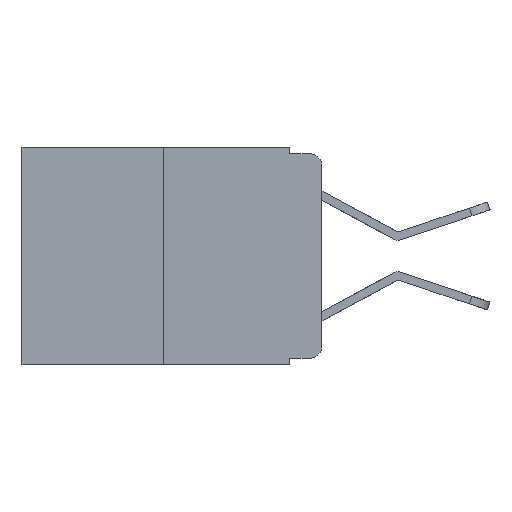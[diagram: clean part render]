
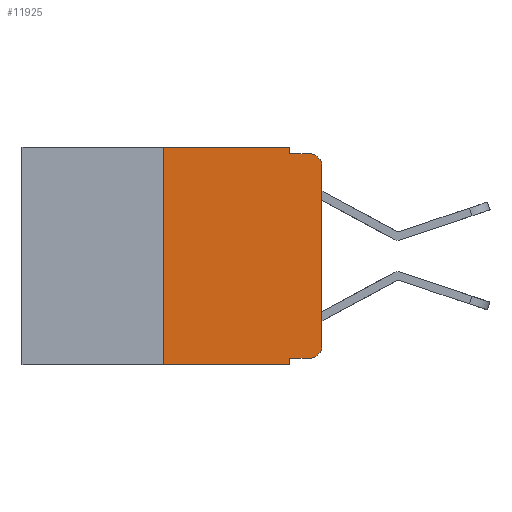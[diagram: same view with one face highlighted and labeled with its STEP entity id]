
A CAD part, left-side view. The second image highlights one B-rep face of the part: STEP entity #11925.
In plain terms, the highlighted planar face has unit normal (-1, 0, 0).
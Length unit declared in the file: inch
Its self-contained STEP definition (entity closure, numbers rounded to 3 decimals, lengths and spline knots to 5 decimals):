
#504 = CARTESIAN_POINT ( 'NONE',  ( 0., 0.02, -0.313 ) ) ;
#676 = DIRECTION ( 'NONE',  ( 0., 0., 1. ) ) ;
#902 = VECTOR ( 'NONE', #6379, 39.37008 ) ;
#942 = LINE ( 'NONE', #8084, #8021 ) ;
#1065 = CARTESIAN_POINT ( 'NONE',  ( 0., 0.051, -0.333 ) ) ;
#1176 = ORIENTED_EDGE ( 'NONE', *, *, #12398, .F. ) ;
#1601 = CARTESIAN_POINT ( 'NONE',  ( 0., 0.25, 0. ) ) ;
#1936 = EDGE_CURVE ( 'NONE', #12264, #3206, #14266, .T. ) ;
#1964 = DIRECTION ( 'NONE',  ( 0., 0., -1. ) ) ;
#2090 = CARTESIAN_POINT ( 'NONE',  ( 0., 0.473, 0. ) ) ;
#2161 = VERTEX_POINT ( 'NONE', #2443 ) ;
#2219 = CIRCLE ( 'NONE', #16954, 0.02 ) ;
#2443 = CARTESIAN_POINT ( 'NONE',  ( 0., 0.051, 0. ) ) ;
#2513 = DIRECTION ( 'NONE',  ( 0., 0., 1. ) ) ;
#2850 = CARTESIAN_POINT ( 'NONE',  ( 0., 0.473, 0. ) ) ;
#2946 = LINE ( 'NONE', #14300, #902 ) ;
#3146 = DIRECTION ( 'NONE',  ( -1., 0., 0. ) ) ;
#3206 = VERTEX_POINT ( 'NONE', #3793 ) ;
#3511 = VERTEX_POINT ( 'NONE', #5145 ) ;
#3548 = VECTOR ( 'NONE', #676, 39.37008 ) ;
#3645 = CARTESIAN_POINT ( 'NONE',  ( 0., 0., -0.313 ) ) ;
#3676 = ORIENTED_EDGE ( 'NONE', *, *, #16733, .T. ) ;
#3783 = VERTEX_POINT ( 'NONE', #1065 ) ;
#3793 = CARTESIAN_POINT ( 'NONE',  ( 0., 0., -0.03 ) ) ;
#4036 = CARTESIAN_POINT ( 'NONE',  ( 0., 0.25, -0.343 ) ) ;
#4244 = AXIS2_PLACEMENT_3D ( 'NONE', #2850, #13674, #5702 ) ;
#4301 = AXIS2_PLACEMENT_3D ( 'NONE', #11351, #3146, #12642 ) ;
#4580 = ORIENTED_EDGE ( 'NONE', *, *, #14122, .F. ) ;
#4705 = VECTOR ( 'NONE', #11730, 39.37008 ) ;
#4884 = VERTEX_POINT ( 'NONE', #9380 ) ;
#5145 = CARTESIAN_POINT ( 'NONE',  ( 0., 0.051, -0.343 ) ) ;
#5265 = LINE ( 'NONE', #12722, #8897 ) ;
#5404 = DIRECTION ( 'NONE',  ( 0., -1., 0. ) ) ;
#5596 = VERTEX_POINT ( 'NONE', #4036 ) ;
#5702 = DIRECTION ( 'NONE',  ( 0., 0., -1. ) ) ;
#5768 = LINE ( 'NONE', #7588, #12460 ) ;
#5895 = ORIENTED_EDGE ( 'NONE', *, *, #11534, .F. ) ;
#6379 = DIRECTION ( 'NONE',  ( 0., -1., 0. ) ) ;
#6737 = CARTESIAN_POINT ( 'NONE',  ( 0., 0., 0. ) ) ;
#7176 = EDGE_CURVE ( 'NONE', #5596, #3511, #2946, .T. ) ;
#7561 = VERTEX_POINT ( 'NONE', #8082 ) ;
#7588 = CARTESIAN_POINT ( 'NONE',  ( 0., 0.051, -0.333 ) ) ;
#7688 = LINE ( 'NONE', #13975, #15090 ) ;
#7963 = EDGE_CURVE ( 'NONE', #7561, #12264, #2219, .T. ) ;
#8014 = EDGE_CURVE ( 'NONE', #16712, #2161, #8785, .T. ) ;
#8021 = VECTOR ( 'NONE', #2513, 39.37008 ) ;
#8082 = CARTESIAN_POINT ( 'NONE',  ( 0., 0.02, -0.333 ) ) ;
#8084 = CARTESIAN_POINT ( 'NONE',  ( 0., 0.25, 0. ) ) ;
#8785 = LINE ( 'NONE', #2090, #4705 ) ;
#8897 = VECTOR ( 'NONE', #10231, 39.37008 ) ;
#9380 = CARTESIAN_POINT ( 'NONE',  ( 0., 0.02, -0.01 ) ) ;
#9775 = EDGE_CURVE ( 'NONE', #3783, #7561, #5768, .T. ) ;
#9985 = VECTOR ( 'NONE', #5404, 39.37008 ) ;
#10231 = DIRECTION ( 'NONE',  ( 0., 0., -1. ) ) ;
#10298 = DIRECTION ( 'NONE',  ( -1., 0., 0. ) ) ;
#10777 = ORIENTED_EDGE ( 'NONE', *, *, #7963, .T. ) ;
#11351 = CARTESIAN_POINT ( 'NONE',  ( 0., 0.02, -0.03 ) ) ;
#11534 = EDGE_CURVE ( 'NONE', #3783, #3511, #5265, .T. ) ;
#11730 = DIRECTION ( 'NONE',  ( 0., -1., 0. ) ) ;
#11786 = ORIENTED_EDGE ( 'NONE', *, *, #8014, .F. ) ;
#11925 = ADVANCED_FACE ( 'NONE', ( #15423 ), #12380, .F. ) ;
#12264 = VERTEX_POINT ( 'NONE', #3645 ) ;
#12380 = PLANE ( 'NONE',  #4244 ) ;
#12398 = EDGE_CURVE ( 'NONE', #5596, #16712, #942, .T. ) ;
#12460 = VECTOR ( 'NONE', #15463, 39.37008 ) ;
#12580 = ORIENTED_EDGE ( 'NONE', *, *, #7176, .T. ) ;
#12642 = DIRECTION ( 'NONE',  ( 0., 0., -1. ) ) ;
#12677 = DIRECTION ( 'NONE',  ( 0., 0., -1. ) ) ;
#12696 = VERTEX_POINT ( 'NONE', #12917 ) ;
#12722 = CARTESIAN_POINT ( 'NONE',  ( 0., 0.051, 0. ) ) ;
#12917 = CARTESIAN_POINT ( 'NONE',  ( 0., 0.051, -0.01 ) ) ;
#13395 = CARTESIAN_POINT ( 'NONE',  ( 0., 0.051, -0.01 ) ) ;
#13437 = LINE ( 'NONE', #13395, #9985 ) ;
#13674 = DIRECTION ( 'NONE',  ( 1., 0., 0. ) ) ;
#13975 = CARTESIAN_POINT ( 'NONE',  ( 0., 0.051, 0. ) ) ;
#14122 = EDGE_CURVE ( 'NONE', #2161, #12696, #7688, .T. ) ;
#14212 = EDGE_LOOP ( 'NONE', ( #17031, #3676, #14395, #4580, #11786, #1176, #12580, #5895, #16428, #10777 ) ) ;
#14266 = LINE ( 'NONE', #6737, #3548 ) ;
#14300 = CARTESIAN_POINT ( 'NONE',  ( 0., 0.473, -0.343 ) ) ;
#14395 = ORIENTED_EDGE ( 'NONE', *, *, #14996, .F. ) ;
#14996 = EDGE_CURVE ( 'NONE', #12696, #4884, #13437, .T. ) ;
#15090 = VECTOR ( 'NONE', #12677, 39.37008 ) ;
#15423 = FACE_OUTER_BOUND ( 'NONE', #14212, .T. ) ;
#15463 = DIRECTION ( 'NONE',  ( 0., -1., 0. ) ) ;
#15608 = CIRCLE ( 'NONE', #4301, 0.02 ) ;
#16428 = ORIENTED_EDGE ( 'NONE', *, *, #9775, .T. ) ;
#16712 = VERTEX_POINT ( 'NONE', #1601 ) ;
#16733 = EDGE_CURVE ( 'NONE', #3206, #4884, #15608, .T. ) ;
#16954 = AXIS2_PLACEMENT_3D ( 'NONE', #504, #10298, #1964 ) ;
#17031 = ORIENTED_EDGE ( 'NONE', *, *, #1936, .T. ) ;
